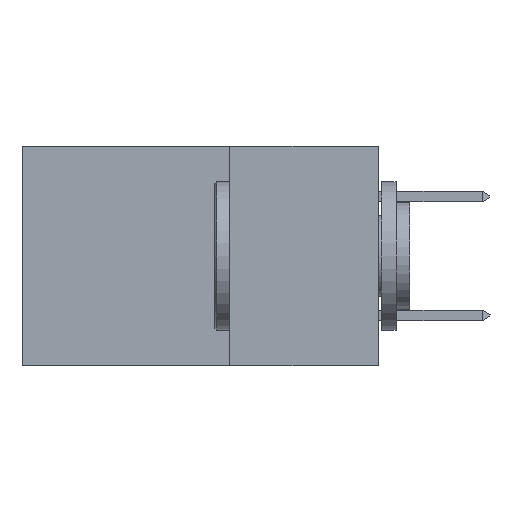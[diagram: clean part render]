
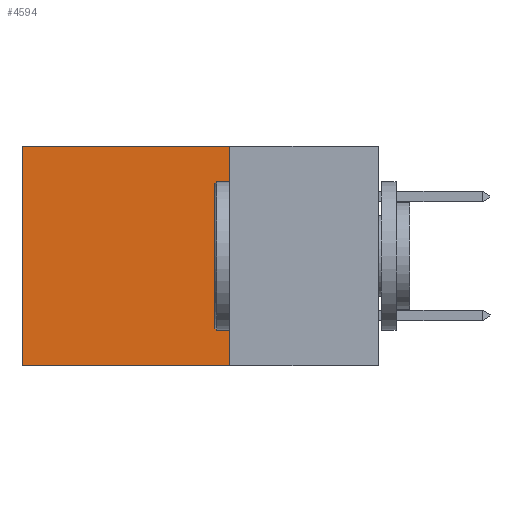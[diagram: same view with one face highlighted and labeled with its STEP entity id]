
A CAD part, left-side view. The second image highlights one B-rep face of the part: STEP entity #4594.
In plain terms, the highlighted planar face has unit normal (-1, 0, 0).
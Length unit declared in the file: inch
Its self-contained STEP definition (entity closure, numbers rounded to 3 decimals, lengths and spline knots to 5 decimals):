
#918 = VERTEX_POINT ( 'NONE', #16689 ) ;
#1261 = CARTESIAN_POINT ( 'NONE',  ( 0.298, 0.25, 0. ) ) ;
#2273 = VECTOR ( 'NONE', #22886, 39.37008 ) ;
#2685 = EDGE_LOOP ( 'NONE', ( #4909, #9341, #18789, #20332 ) ) ;
#3466 = AXIS2_PLACEMENT_3D ( 'NONE', #1261, #19629, #8634 ) ;
#3907 = FACE_OUTER_BOUND ( 'NONE', #2685, .T. ) ;
#4030 = VERTEX_POINT ( 'NONE', #25497 ) ;
#4078 = LINE ( 'NONE', #13143, #21133 ) ;
#4594 = ADVANCED_FACE ( 'NONE', ( #3907 ), #25025, .F. ) ;
#4909 = ORIENTED_EDGE ( 'NONE', *, *, #5700, .T. ) ;
#5631 = LINE ( 'NONE', #24053, #22648 ) ;
#5700 = EDGE_CURVE ( 'NONE', #6160, #4030, #5631, .T. ) ;
#6160 = VERTEX_POINT ( 'NONE', #8681 ) ;
#8634 = DIRECTION ( 'NONE',  ( 0., 0., -1. ) ) ;
#8681 = CARTESIAN_POINT ( 'NONE',  ( 0.298, 0.6, 0. ) ) ;
#9341 = ORIENTED_EDGE ( 'NONE', *, *, #24603, .F. ) ;
#9591 = VECTOR ( 'NONE', #23547, 39.37008 ) ;
#10789 = VERTEX_POINT ( 'NONE', #11678 ) ;
#11678 = CARTESIAN_POINT ( 'NONE',  ( 0.298, 0.25, -0.37 ) ) ;
#13143 = CARTESIAN_POINT ( 'NONE',  ( 0.298, 0.25, 0. ) ) ;
#14279 = LINE ( 'NONE', #16402, #2273 ) ;
#16402 = CARTESIAN_POINT ( 'NONE',  ( 0.298, 0.25, -0.37 ) ) ;
#16689 = CARTESIAN_POINT ( 'NONE',  ( 0.298, 0.25, 0. ) ) ;
#16979 = EDGE_CURVE ( 'NONE', #918, #10789, #21976, .T. ) ;
#18789 = ORIENTED_EDGE ( 'NONE', *, *, #16979, .F. ) ;
#19629 = DIRECTION ( 'NONE',  ( 1., 0., 0. ) ) ;
#20332 = ORIENTED_EDGE ( 'NONE', *, *, #20657, .T. ) ;
#20657 = EDGE_CURVE ( 'NONE', #918, #6160, #4078, .T. ) ;
#21133 = VECTOR ( 'NONE', #26236, 39.37008 ) ;
#21976 = LINE ( 'NONE', #25740, #9591 ) ;
#22648 = VECTOR ( 'NONE', #24086, 39.37008 ) ;
#22886 = DIRECTION ( 'NONE',  ( 0., 1., 0. ) ) ;
#23547 = DIRECTION ( 'NONE',  ( 0., 0., -1. ) ) ;
#24053 = CARTESIAN_POINT ( 'NONE',  ( 0.298, 0.6, 0. ) ) ;
#24086 = DIRECTION ( 'NONE',  ( 0., 0., -1. ) ) ;
#24603 = EDGE_CURVE ( 'NONE', #10789, #4030, #14279, .T. ) ;
#25025 = PLANE ( 'NONE',  #3466 ) ;
#25497 = CARTESIAN_POINT ( 'NONE',  ( 0.298, 0.6, -0.37 ) ) ;
#25740 = CARTESIAN_POINT ( 'NONE',  ( 0.298, 0.25, 0. ) ) ;
#26236 = DIRECTION ( 'NONE',  ( 0., 1., 0. ) ) ;
